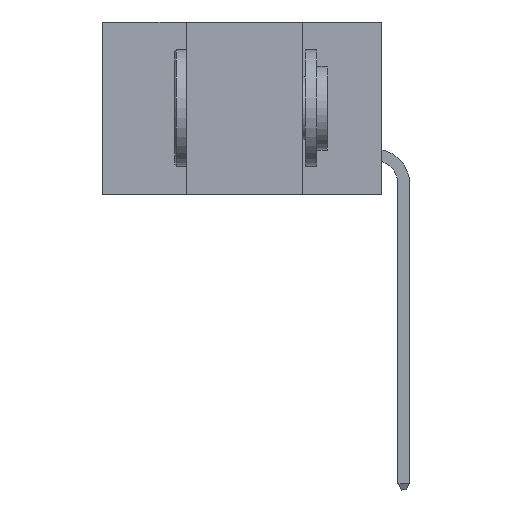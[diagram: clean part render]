
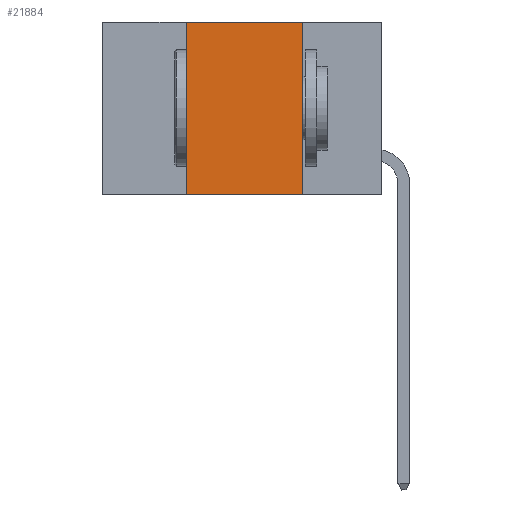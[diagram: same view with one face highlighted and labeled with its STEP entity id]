
A CAD part, left-side view. The second image highlights one B-rep face of the part: STEP entity #21884.
In plain terms, the highlighted planar face has unit normal (-1, 0, 0).
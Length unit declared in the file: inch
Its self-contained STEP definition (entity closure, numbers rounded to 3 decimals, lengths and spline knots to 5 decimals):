
#139 = VECTOR ( 'NONE', #10003, 39.37008 ) ;
#808 = FACE_OUTER_BOUND ( 'NONE', #12588, .T. ) ;
#2266 = VERTEX_POINT ( 'NONE', #20277 ) ;
#2269 = EDGE_CURVE ( 'NONE', #9467, #15088, #24249, .T. ) ;
#2415 = EDGE_CURVE ( 'NONE', #2266, #22579, #13826, .T. ) ;
#2474 = CARTESIAN_POINT ( 'NONE',  ( 0., 0.6, -0.37 ) ) ;
#5193 = EDGE_CURVE ( 'NONE', #15088, #2266, #20983, .T. ) ;
#5308 = DIRECTION ( 'NONE',  ( 0., 0., -1. ) ) ;
#5932 = ORIENTED_EDGE ( 'NONE', *, *, #2269, .F. ) ;
#5936 = CARTESIAN_POINT ( 'NONE',  ( 0., 0.42, 0. ) ) ;
#7211 = LINE ( 'NONE', #2474, #18924 ) ;
#8857 = ORIENTED_EDGE ( 'NONE', *, *, #2415, .F. ) ;
#9467 = VERTEX_POINT ( 'NONE', #19836 ) ;
#10003 = DIRECTION ( 'NONE',  ( 0., 0., 1. ) ) ;
#12588 = EDGE_LOOP ( 'NONE', ( #8857, #16641, #5932, #13247 ) ) ;
#13247 = ORIENTED_EDGE ( 'NONE', *, *, #19260, .T. ) ;
#13430 = AXIS2_PLACEMENT_3D ( 'NONE', #23934, #19911, #5308 ) ;
#13826 = LINE ( 'NONE', #16219, #25521 ) ;
#13939 = DIRECTION ( 'NONE',  ( 0., 0., -1. ) ) ;
#15088 = VERTEX_POINT ( 'NONE', #22415 ) ;
#16219 = CARTESIAN_POINT ( 'NONE',  ( 0., 0.17, 0. ) ) ;
#16641 = ORIENTED_EDGE ( 'NONE', *, *, #5193, .F. ) ;
#17096 = VECTOR ( 'NONE', #17257, 39.37008 ) ;
#17257 = DIRECTION ( 'NONE',  ( 0., -1., 0. ) ) ;
#18924 = VECTOR ( 'NONE', #23280, 39.37008 ) ;
#19260 = EDGE_CURVE ( 'NONE', #9467, #22579, #7211, .T. ) ;
#19826 = PLANE ( 'NONE',  #13430 ) ;
#19836 = CARTESIAN_POINT ( 'NONE',  ( 0., 0.42, -0.37 ) ) ;
#19911 = DIRECTION ( 'NONE',  ( 1., 0., 0. ) ) ;
#20277 = CARTESIAN_POINT ( 'NONE',  ( 0., 0.17, 0. ) ) ;
#20983 = LINE ( 'NONE', #23536, #17096 ) ;
#21884 = ADVANCED_FACE ( 'NONE', ( #808 ), #19826, .F. ) ;
#22415 = CARTESIAN_POINT ( 'NONE',  ( 0., 0.42, 0. ) ) ;
#22579 = VERTEX_POINT ( 'NONE', #26485 ) ;
#23280 = DIRECTION ( 'NONE',  ( 0., -1., 0. ) ) ;
#23536 = CARTESIAN_POINT ( 'NONE',  ( 0., 0.6, 0. ) ) ;
#23934 = CARTESIAN_POINT ( 'NONE',  ( 0., 0.6, 0. ) ) ;
#24249 = LINE ( 'NONE', #5936, #139 ) ;
#25521 = VECTOR ( 'NONE', #13939, 39.37008 ) ;
#26485 = CARTESIAN_POINT ( 'NONE',  ( 0., 0.17, -0.37 ) ) ;
